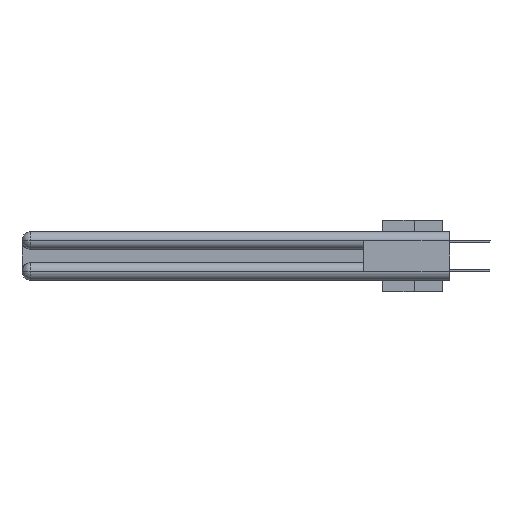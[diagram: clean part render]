
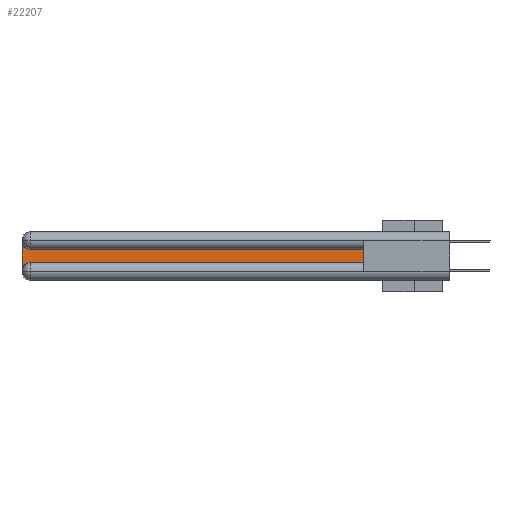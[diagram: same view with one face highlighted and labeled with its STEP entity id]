
A CAD part, left-side view. The second image highlights one B-rep face of the part: STEP entity #22207.
In plain terms, the highlighted planar face has unit normal (-1, 0, 0).
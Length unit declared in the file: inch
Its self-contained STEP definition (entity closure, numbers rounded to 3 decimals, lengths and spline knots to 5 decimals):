
#641 = ORIENTED_EDGE ( 'NONE', *, *, #6747, .T. ) ;
#1043 = CARTESIAN_POINT ( 'NONE',  ( 0.075, 0.6, -0.2175 ) ) ;
#1436 = DIRECTION ( 'NONE',  ( 0., -1., 0. ) ) ;
#1458 = VERTEX_POINT ( 'NONE', #6129 ) ;
#2557 = VERTEX_POINT ( 'NONE', #26820 ) ;
#3048 = VECTOR ( 'NONE', #8479, 39.37008 ) ;
#3152 = CIRCLE ( 'NONE', #27534, 0.06 ) ;
#3886 = CARTESIAN_POINT ( 'NONE',  ( 0.075, 0.6, -0.2175 ) ) ;
#6129 = CARTESIAN_POINT ( 'NONE',  ( 0.075, 3., -0.0625 ) ) ;
#6747 = EDGE_CURVE ( 'NONE', #10315, #26614, #9061, .T. ) ;
#7504 = FACE_OUTER_BOUND ( 'NONE', #25188, .T. ) ;
#8113 = LINE ( 'NONE', #28094, #20522 ) ;
#8479 = DIRECTION ( 'NONE',  ( 0., 1., 0. ) ) ;
#8743 = DIRECTION ( 'NONE',  ( 0., 0., -1. ) ) ;
#9061 = LINE ( 'NONE', #31405, #11483 ) ;
#9999 = EDGE_CURVE ( 'NONE', #1458, #32492, #8113, .T. ) ;
#10115 = DIRECTION ( 'NONE',  ( 0., 0., -1. ) ) ;
#10148 = CARTESIAN_POINT ( 'NONE',  ( 0.075, 3., -0.1225 ) ) ;
#10315 = VERTEX_POINT ( 'NONE', #1043 ) ;
#10468 = CIRCLE ( 'NONE', #18700, 0.06 ) ;
#10663 = CARTESIAN_POINT ( 'NONE',  ( 0.075, 2.94, -0.2775 ) ) ;
#11402 = LINE ( 'NONE', #3886, #17049 ) ;
#11483 = VECTOR ( 'NONE', #26598, 39.37008 ) ;
#13040 = ORIENTED_EDGE ( 'NONE', *, *, #30101, .T. ) ;
#13228 = DIRECTION ( 'NONE',  ( 0., 0., -1. ) ) ;
#13667 = ORIENTED_EDGE ( 'NONE', *, *, #16404, .T. ) ;
#13893 = CARTESIAN_POINT ( 'NONE',  ( 0.075, 2.94, -0.0625 ) ) ;
#14972 = PLANE ( 'NONE',  #21574 ) ;
#15201 = DIRECTION ( 'NONE',  ( 0., 0., -1. ) ) ;
#16404 = EDGE_CURVE ( 'NONE', #32492, #32023, #10468, .T. ) ;
#17049 = VECTOR ( 'NONE', #1436, 39.37008 ) ;
#17053 = ORIENTED_EDGE ( 'NONE', *, *, #30470, .T. ) ;
#17476 = CARTESIAN_POINT ( 'NONE',  ( 0.075, 2.94, -0.2175 ) ) ;
#18700 = AXIS2_PLACEMENT_3D ( 'NONE', #10663, #28533, #13228 ) ;
#19595 = CARTESIAN_POINT ( 'NONE',  ( 0.075, 0.6, -0.1225 ) ) ;
#20522 = VECTOR ( 'NONE', #10115, 39.37008 ) ;
#21126 = CARTESIAN_POINT ( 'NONE',  ( 0.075, 0.6, -0.1225 ) ) ;
#21168 = DIRECTION ( 'NONE',  ( 1., 0., 0. ) ) ;
#21294 = EDGE_CURVE ( 'NONE', #2557, #1458, #3152, .T. ) ;
#21574 = AXIS2_PLACEMENT_3D ( 'NONE', #10148, #25322, #15201 ) ;
#22207 = ADVANCED_FACE ( 'NONE', ( #7504 ), #14972, .F. ) ;
#23445 = LINE ( 'NONE', #21126, #3048 ) ;
#25188 = EDGE_LOOP ( 'NONE', ( #13040, #26963, #31485, #13667, #17053, #641 ) ) ;
#25322 = DIRECTION ( 'NONE',  ( 1., 0., 0. ) ) ;
#26598 = DIRECTION ( 'NONE',  ( 0., 0., 1. ) ) ;
#26614 = VERTEX_POINT ( 'NONE', #19595 ) ;
#26820 = CARTESIAN_POINT ( 'NONE',  ( 0.075, 2.94, -0.1225 ) ) ;
#26963 = ORIENTED_EDGE ( 'NONE', *, *, #21294, .T. ) ;
#27534 = AXIS2_PLACEMENT_3D ( 'NONE', #13893, #21168, #8743 ) ;
#28094 = CARTESIAN_POINT ( 'NONE',  ( 0.075, 3., -0.2175 ) ) ;
#28533 = DIRECTION ( 'NONE',  ( 1., 0., 0. ) ) ;
#30022 = CARTESIAN_POINT ( 'NONE',  ( 0.075, 3., -0.2775 ) ) ;
#30101 = EDGE_CURVE ( 'NONE', #26614, #2557, #23445, .T. ) ;
#30470 = EDGE_CURVE ( 'NONE', #32023, #10315, #11402, .T. ) ;
#31405 = CARTESIAN_POINT ( 'NONE',  ( 0.075, 0.6, -0.2175 ) ) ;
#31485 = ORIENTED_EDGE ( 'NONE', *, *, #9999, .T. ) ;
#32023 = VERTEX_POINT ( 'NONE', #17476 ) ;
#32492 = VERTEX_POINT ( 'NONE', #30022 ) ;
